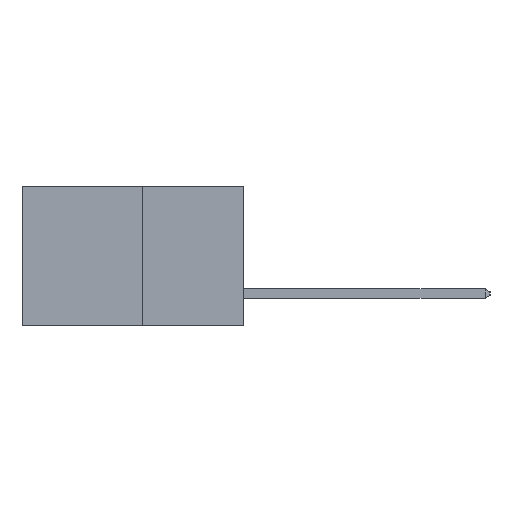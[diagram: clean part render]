
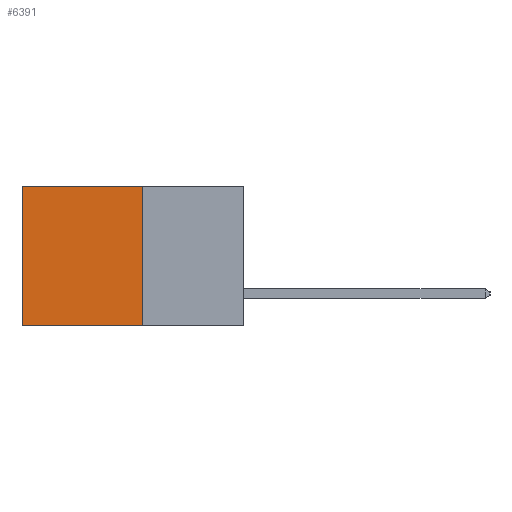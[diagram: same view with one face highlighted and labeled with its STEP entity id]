
A CAD part, left-side view. The second image highlights one B-rep face of the part: STEP entity #6391.
In plain terms, the highlighted planar face has unit normal (-1, 0, 0).
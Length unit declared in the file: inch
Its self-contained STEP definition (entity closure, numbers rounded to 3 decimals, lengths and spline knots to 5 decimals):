
#4 = EDGE_CURVE ( 'NONE', #3196, #6241, #6235, .T. ) ;
#184 = ORIENTED_EDGE ( 'NONE', *, *, #5733, .T. ) ;
#357 = DIRECTION ( 'NONE',  ( 0., 0., -1. ) ) ;
#770 = AXIS2_PLACEMENT_3D ( 'NONE', #3163, #1441, #1359 ) ;
#1035 = CARTESIAN_POINT ( 'NONE',  ( 0.277, 0.27, 0. ) ) ;
#1359 = DIRECTION ( 'NONE',  ( 0., 0., -1. ) ) ;
#1441 = DIRECTION ( 'NONE',  ( 1., 0., 0. ) ) ;
#1627 = ORIENTED_EDGE ( 'NONE', *, *, #4, .F. ) ;
#1875 = LINE ( 'NONE', #3321, #3416 ) ;
#1926 = CARTESIAN_POINT ( 'NONE',  ( 0.277, 0.59, -0.37 ) ) ;
#1937 = ORIENTED_EDGE ( 'NONE', *, *, #2672, .F. ) ;
#2560 = DIRECTION ( 'NONE',  ( 0., 1., 0. ) ) ;
#2631 = VECTOR ( 'NONE', #2560, 39.37008 ) ;
#2672 = EDGE_CURVE ( 'NONE', #6241, #5354, #7708, .T. ) ;
#3001 = EDGE_CURVE ( 'NONE', #3196, #4648, #8066, .T. ) ;
#3163 = CARTESIAN_POINT ( 'NONE',  ( 0.277, 0.27, -0.37 ) ) ;
#3196 = VERTEX_POINT ( 'NONE', #1035 ) ;
#3321 = CARTESIAN_POINT ( 'NONE',  ( 0.277, 0.59, -0.37 ) ) ;
#3416 = VECTOR ( 'NONE', #4664, 39.37008 ) ;
#3911 = CARTESIAN_POINT ( 'NONE',  ( 0.277, 0.27, -0.37 ) ) ;
#4036 = EDGE_LOOP ( 'NONE', ( #184, #1937, #1627, #5168 ) ) ;
#4648 = VERTEX_POINT ( 'NONE', #6172 ) ;
#4664 = DIRECTION ( 'NONE',  ( 0., 0., -1. ) ) ;
#4666 = PLANE ( 'NONE',  #770 ) ;
#5168 = ORIENTED_EDGE ( 'NONE', *, *, #3001, .T. ) ;
#5354 = VERTEX_POINT ( 'NONE', #1926 ) ;
#5480 = CARTESIAN_POINT ( 'NONE',  ( 0.277, 0.27, 0. ) ) ;
#5733 = EDGE_CURVE ( 'NONE', #4648, #5354, #1875, .T. ) ;
#5827 = DIRECTION ( 'NONE',  ( 0., 1., 0. ) ) ;
#6156 = VECTOR ( 'NONE', #5827, 39.37008 ) ;
#6172 = CARTESIAN_POINT ( 'NONE',  ( 0.277, 0.59, 0. ) ) ;
#6235 = LINE ( 'NONE', #3911, #8126 ) ;
#6241 = VERTEX_POINT ( 'NONE', #7219 ) ;
#6391 = ADVANCED_FACE ( 'NONE', ( #7769 ), #4666, .F. ) ;
#7219 = CARTESIAN_POINT ( 'NONE',  ( 0.277, 0.27, -0.37 ) ) ;
#7454 = CARTESIAN_POINT ( 'NONE',  ( 0.277, 0.27, -0.37 ) ) ;
#7708 = LINE ( 'NONE', #7454, #2631 ) ;
#7769 = FACE_OUTER_BOUND ( 'NONE', #4036, .T. ) ;
#8066 = LINE ( 'NONE', #5480, #6156 ) ;
#8126 = VECTOR ( 'NONE', #357, 39.37008 ) ;
